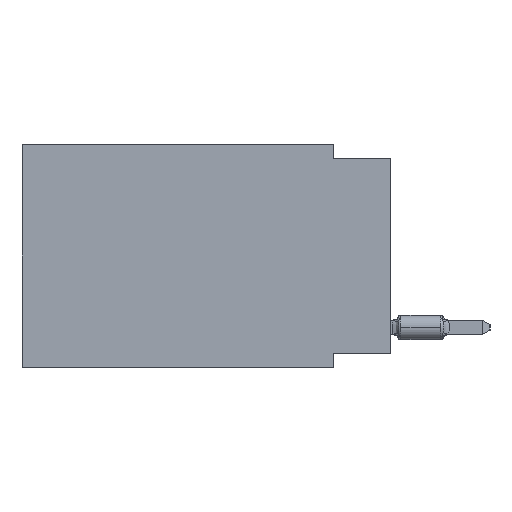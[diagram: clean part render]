
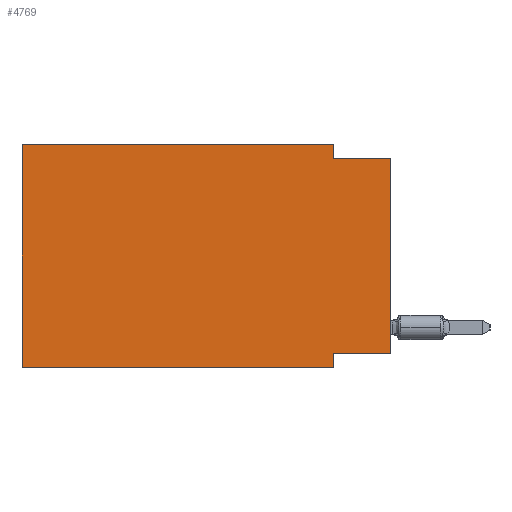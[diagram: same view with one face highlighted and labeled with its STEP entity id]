
A CAD part, left-side view. The second image highlights one B-rep face of the part: STEP entity #4769.
In plain terms, the highlighted planar face has unit normal (-1, 0, 0).
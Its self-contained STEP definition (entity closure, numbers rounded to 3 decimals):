
#416 = ORIENTED_EDGE ( 'NONE', *, *, #37788, .T. ) ;
#610 = CARTESIAN_POINT ( 'NONE',  ( 0., 2.54, -9.906 ) ) ;
#826 = LINE ( 'NONE', #27315, #37682 ) ;
#1265 = ORIENTED_EDGE ( 'NONE', *, *, #37346, .T. ) ;
#1734 = DIRECTION ( 'NONE',  ( 0., -1., 0. ) ) ;
#1788 = CARTESIAN_POINT ( 'NONE',  ( 0., 0., 0. ) ) ;
#2293 = EDGE_CURVE ( 'NONE', #26064, #15369, #22896, .T. ) ;
#2357 = LINE ( 'NONE', #14123, #30337 ) ;
#2826 = ORIENTED_EDGE ( 'NONE', *, *, #15886, .F. ) ;
#4096 = CARTESIAN_POINT ( 'NONE',  ( 0., 0., -9.271 ) ) ;
#4309 = CARTESIAN_POINT ( 'NONE',  ( 0., 0., -0.635 ) ) ;
#4769 = ADVANCED_FACE ( 'NONE', ( #30017 ), #12737, .F. ) ;
#6313 = LINE ( 'NONE', #610, #33304 ) ;
#9200 = LINE ( 'NONE', #12513, #14607 ) ;
#9374 = VERTEX_POINT ( 'NONE', #4096 ) ;
#9865 = VERTEX_POINT ( 'NONE', #17129 ) ;
#10330 = CARTESIAN_POINT ( 'NONE',  ( 0., 0., -0.635 ) ) ;
#11180 = LINE ( 'NONE', #1788, #37923 ) ;
#12021 = VECTOR ( 'NONE', #27653, 1000. ) ;
#12513 = CARTESIAN_POINT ( 'NONE',  ( 0., 16.383, 0. ) ) ;
#12737 = PLANE ( 'NONE',  #32073 ) ;
#13744 = DIRECTION ( 'NONE',  ( 0., 0., 1. ) ) ;
#14123 = CARTESIAN_POINT ( 'NONE',  ( 0., 16.383, 0. ) ) ;
#14184 = CARTESIAN_POINT ( 'NONE',  ( 0., 2.54, 0. ) ) ;
#14607 = VECTOR ( 'NONE', #27834, 1000. ) ;
#15369 = VERTEX_POINT ( 'NONE', #10330 ) ;
#15487 = CARTESIAN_POINT ( 'NONE',  ( 0., 16.383, 0. ) ) ;
#15886 = EDGE_CURVE ( 'NONE', #18359, #26018, #6313, .T. ) ;
#16669 = EDGE_CURVE ( 'NONE', #9374, #18359, #18919, .T. ) ;
#17129 = CARTESIAN_POINT ( 'NONE',  ( 0., 16.383, 0. ) ) ;
#17412 = VERTEX_POINT ( 'NONE', #24876 ) ;
#18359 = VERTEX_POINT ( 'NONE', #38551 ) ;
#18490 = EDGE_CURVE ( 'NONE', #32494, #26064, #36721, .T. ) ;
#18579 = CARTESIAN_POINT ( 'NONE',  ( 0., 2.54, -0.635 ) ) ;
#18874 = DIRECTION ( 'NONE',  ( 0., -1., 0. ) ) ;
#18919 = LINE ( 'NONE', #30907, #21407 ) ;
#20001 = EDGE_LOOP ( 'NONE', ( #1265, #32035, #35627, #38428, #34871, #416, #2826, #30348 ) ) ;
#20166 = EDGE_CURVE ( 'NONE', #17412, #9865, #2357, .T. ) ;
#21407 = VECTOR ( 'NONE', #25191, 1000. ) ;
#22896 = LINE ( 'NONE', #4309, #30067 ) ;
#24498 = DIRECTION ( 'NONE',  ( 1., 0., 0. ) ) ;
#24876 = CARTESIAN_POINT ( 'NONE',  ( 0., 16.383, -9.906 ) ) ;
#25191 = DIRECTION ( 'NONE',  ( 0., 1., 0. ) ) ;
#26018 = VERTEX_POINT ( 'NONE', #33753 ) ;
#26064 = VERTEX_POINT ( 'NONE', #18579 ) ;
#27272 = CARTESIAN_POINT ( 'NONE',  ( 0., 2.54, 0. ) ) ;
#27315 = CARTESIAN_POINT ( 'NONE',  ( 0., 16.383, -9.906 ) ) ;
#27653 = DIRECTION ( 'NONE',  ( 0., 0., -1. ) ) ;
#27834 = DIRECTION ( 'NONE',  ( 0., -1., 0. ) ) ;
#30017 = FACE_OUTER_BOUND ( 'NONE', #20001, .T. ) ;
#30067 = VECTOR ( 'NONE', #1734, 1000. ) ;
#30337 = VECTOR ( 'NONE', #38461, 1000. ) ;
#30348 = ORIENTED_EDGE ( 'NONE', *, *, #16669, .F. ) ;
#30907 = CARTESIAN_POINT ( 'NONE',  ( 0., 0., -9.271 ) ) ;
#31733 = EDGE_CURVE ( 'NONE', #9865, #32494, #9200, .T. ) ;
#32035 = ORIENTED_EDGE ( 'NONE', *, *, #2293, .F. ) ;
#32073 = AXIS2_PLACEMENT_3D ( 'NONE', #15487, #24498, #33351 ) ;
#32494 = VERTEX_POINT ( 'NONE', #14184 ) ;
#33304 = VECTOR ( 'NONE', #35741, 1000. ) ;
#33351 = DIRECTION ( 'NONE',  ( 0., 0., -1. ) ) ;
#33753 = CARTESIAN_POINT ( 'NONE',  ( 0., 2.54, -9.906 ) ) ;
#34871 = ORIENTED_EDGE ( 'NONE', *, *, #20166, .F. ) ;
#35627 = ORIENTED_EDGE ( 'NONE', *, *, #18490, .F. ) ;
#35741 = DIRECTION ( 'NONE',  ( 0., 0., -1. ) ) ;
#36721 = LINE ( 'NONE', #27272, #12021 ) ;
#37346 = EDGE_CURVE ( 'NONE', #9374, #15369, #11180, .T. ) ;
#37682 = VECTOR ( 'NONE', #18874, 1000. ) ;
#37788 = EDGE_CURVE ( 'NONE', #17412, #26018, #826, .T. ) ;
#37923 = VECTOR ( 'NONE', #13744, 1000. ) ;
#38428 = ORIENTED_EDGE ( 'NONE', *, *, #31733, .F. ) ;
#38461 = DIRECTION ( 'NONE',  ( 0., 0., 1. ) ) ;
#38551 = CARTESIAN_POINT ( 'NONE',  ( 0., 2.54, -9.271 ) ) ;
